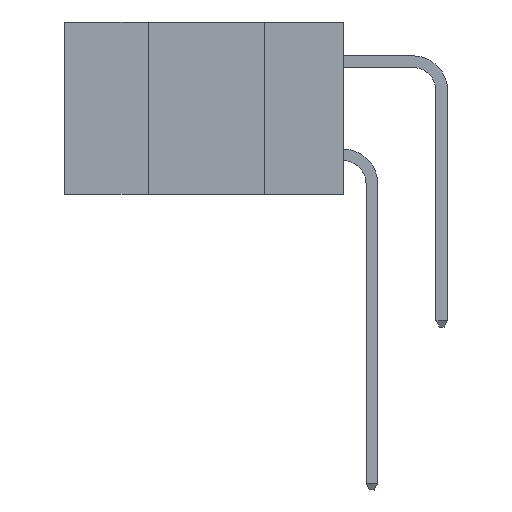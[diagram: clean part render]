
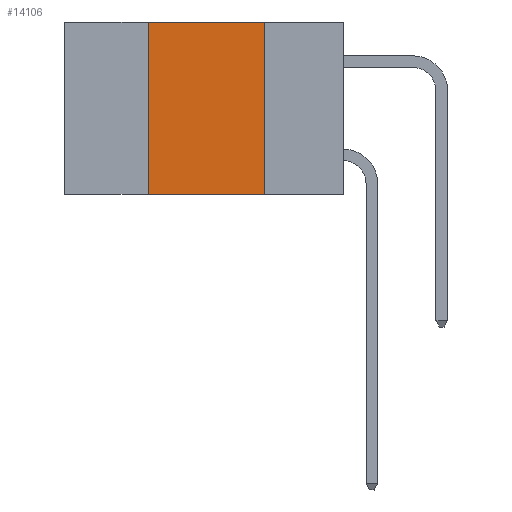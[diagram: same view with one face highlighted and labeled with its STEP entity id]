
A CAD part, left-side view. The second image highlights one B-rep face of the part: STEP entity #14106.
In plain terms, the highlighted planar face has unit normal (-1, 0, 0).
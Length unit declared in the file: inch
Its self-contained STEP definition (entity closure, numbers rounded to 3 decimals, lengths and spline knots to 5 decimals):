
#216 = DIRECTION ( 'NONE',  ( 0., 0., -1. ) ) ;
#495 = CARTESIAN_POINT ( 'NONE',  ( 0., 0.6, 0. ) ) ;
#499 = ORIENTED_EDGE ( 'NONE', *, *, #16742, .F. ) ;
#636 = VERTEX_POINT ( 'NONE', #3198 ) ;
#1156 = DIRECTION ( 'NONE',  ( 0., -1., 0. ) ) ;
#2656 = VERTEX_POINT ( 'NONE', #9421 ) ;
#2665 = CARTESIAN_POINT ( 'NONE',  ( 0., 0.17, -0.37 ) ) ;
#2937 = VERTEX_POINT ( 'NONE', #2665 ) ;
#3198 = CARTESIAN_POINT ( 'NONE',  ( 0., 0.17, 0. ) ) ;
#3212 = EDGE_LOOP ( 'NONE', ( #13134, #499, #4194, #18160 ) ) ;
#4194 = ORIENTED_EDGE ( 'NONE', *, *, #12438, .F. ) ;
#4283 = DIRECTION ( 'NONE',  ( 1., 0., 0. ) ) ;
#4345 = CARTESIAN_POINT ( 'NONE',  ( 0., 0.6, 0. ) ) ;
#5138 = VECTOR ( 'NONE', #5860, 39.37008 ) ;
#5726 = VECTOR ( 'NONE', #13924, 39.37008 ) ;
#5860 = DIRECTION ( 'NONE',  ( 0., -1., 0. ) ) ;
#6002 = LINE ( 'NONE', #495, #5138 ) ;
#7039 = CARTESIAN_POINT ( 'NONE',  ( 0., 0.42, 0. ) ) ;
#8090 = LINE ( 'NONE', #8213, #15124 ) ;
#8213 = CARTESIAN_POINT ( 'NONE',  ( 0., 0.6, -0.37 ) ) ;
#8508 = PLANE ( 'NONE',  #9761 ) ;
#8952 = CARTESIAN_POINT ( 'NONE',  ( 0., 0.17, 0. ) ) ;
#9421 = CARTESIAN_POINT ( 'NONE',  ( 0., 0.42, -0.37 ) ) ;
#9497 = EDGE_CURVE ( 'NONE', #636, #2937, #15723, .T. ) ;
#9670 = CARTESIAN_POINT ( 'NONE',  ( 0., 0.42, 0. ) ) ;
#9761 = AXIS2_PLACEMENT_3D ( 'NONE', #4345, #4283, #216 ) ;
#11694 = DIRECTION ( 'NONE',  ( 0., 0., -1. ) ) ;
#12438 = EDGE_CURVE ( 'NONE', #2656, #14227, #13438, .T. ) ;
#13134 = ORIENTED_EDGE ( 'NONE', *, *, #9497, .F. ) ;
#13438 = LINE ( 'NONE', #9670, #5726 ) ;
#13746 = VECTOR ( 'NONE', #11694, 39.37008 ) ;
#13924 = DIRECTION ( 'NONE',  ( 0., 0., 1. ) ) ;
#14053 = EDGE_CURVE ( 'NONE', #2656, #2937, #8090, .T. ) ;
#14106 = ADVANCED_FACE ( 'NONE', ( #16013 ), #8508, .F. ) ;
#14227 = VERTEX_POINT ( 'NONE', #7039 ) ;
#15124 = VECTOR ( 'NONE', #1156, 39.37008 ) ;
#15723 = LINE ( 'NONE', #8952, #13746 ) ;
#16013 = FACE_OUTER_BOUND ( 'NONE', #3212, .T. ) ;
#16742 = EDGE_CURVE ( 'NONE', #14227, #636, #6002, .T. ) ;
#18160 = ORIENTED_EDGE ( 'NONE', *, *, #14053, .T. ) ;
